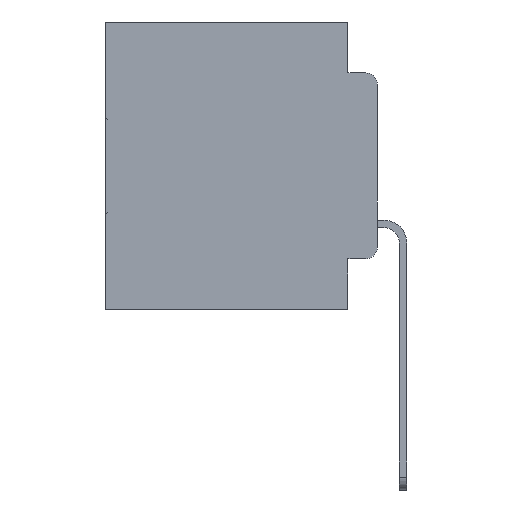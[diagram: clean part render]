
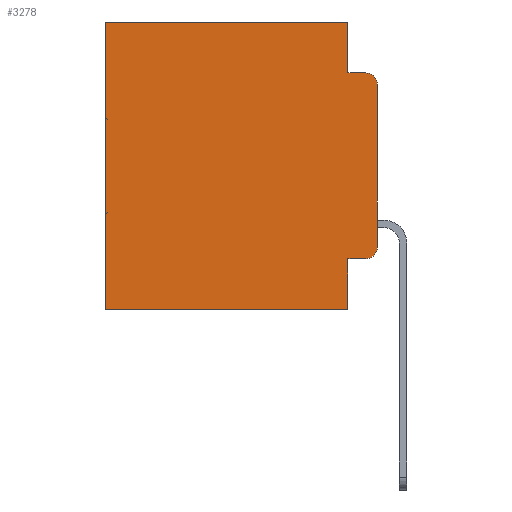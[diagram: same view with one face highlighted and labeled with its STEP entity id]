
A CAD part, left-side view. The second image highlights one B-rep face of the part: STEP entity #3278.
In plain terms, the highlighted planar face has unit normal (-1, 0, 0).
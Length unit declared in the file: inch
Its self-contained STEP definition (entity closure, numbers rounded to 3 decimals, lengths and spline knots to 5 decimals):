
#520 = DIRECTION ( 'NONE',  ( 0., 1., 0. ) ) ;
#866 = ORIENTED_EDGE ( 'NONE', *, *, #29314, .T. ) ;
#1343 = ORIENTED_EDGE ( 'NONE', *, *, #12030, .T. ) ;
#1952 = LINE ( 'NONE', #20739, #21634 ) ;
#2817 = CARTESIAN_POINT ( 'NONE',  ( 0.298, 0., 0. ) ) ;
#3278 = ADVANCED_FACE ( 'NONE', ( #25353 ), #19009, .F. ) ;
#3777 = CARTESIAN_POINT ( 'NONE',  ( 0.298, 0.02, -0.3915 ) ) ;
#4043 = ORIENTED_EDGE ( 'NONE', *, *, #12696, .F. ) ;
#4755 = ORIENTED_EDGE ( 'NONE', *, *, #29872, .F. ) ;
#5455 = CARTESIAN_POINT ( 'NONE',  ( 0.298, 0.051, 0. ) ) ;
#5644 = CARTESIAN_POINT ( 'NONE',  ( 0.298, 0.473, -0.5 ) ) ;
#6081 = VECTOR ( 'NONE', #30742, 39.37008 ) ;
#6240 = CARTESIAN_POINT ( 'NONE',  ( 0.298, 0., 0. ) ) ;
#6361 = DIRECTION ( 'NONE',  ( 0., 0., -1. ) ) ;
#6434 = LINE ( 'NONE', #2817, #7291 ) ;
#6481 = DIRECTION ( 'NONE',  ( 0., 0., -1. ) ) ;
#6741 = LINE ( 'NONE', #5455, #20157 ) ;
#7291 = VECTOR ( 'NONE', #20728, 39.37008 ) ;
#7894 = VERTEX_POINT ( 'NONE', #5644 ) ;
#8541 = VERTEX_POINT ( 'NONE', #19485 ) ;
#9896 = ORIENTED_EDGE ( 'NONE', *, *, #18399, .F. ) ;
#10313 = ORIENTED_EDGE ( 'NONE', *, *, #21648, .F. ) ;
#11189 = EDGE_CURVE ( 'NONE', #12075, #28483, #6434, .T. ) ;
#11825 = AXIS2_PLACEMENT_3D ( 'NONE', #6240, #21447, #6361 ) ;
#12024 = CARTESIAN_POINT ( 'NONE',  ( 0.298, 0.02, -0.1085 ) ) ;
#12030 = EDGE_CURVE ( 'NONE', #28483, #7894, #20564, .T. ) ;
#12075 = VERTEX_POINT ( 'NONE', #19070 ) ;
#12534 = LINE ( 'NONE', #13704, #31058 ) ;
#12696 = EDGE_CURVE ( 'NONE', #20193, #7894, #16787, .T. ) ;
#13370 = CARTESIAN_POINT ( 'NONE',  ( 0.298, 0.051, -0.5 ) ) ;
#13704 = CARTESIAN_POINT ( 'NONE',  ( 0.298, 0.051, 0. ) ) ;
#13837 = LINE ( 'NONE', #28328, #6081 ) ;
#14488 = DIRECTION ( 'NONE',  ( 0., 0., -1. ) ) ;
#14734 = EDGE_LOOP ( 'NONE', ( #27144, #866, #9896, #10313, #32414, #1343, #4043, #4755, #22200, #31221 ) ) ;
#15334 = EDGE_CURVE ( 'NONE', #8541, #15939, #1952, .T. ) ;
#15595 = VECTOR ( 'NONE', #18859, 39.37008 ) ;
#15907 = CARTESIAN_POINT ( 'NONE',  ( 0.298, 0.02, -0.0885 ) ) ;
#15939 = VERTEX_POINT ( 'NONE', #27233 ) ;
#16166 = DIRECTION ( 'NONE',  ( 0., 0., -1. ) ) ;
#16174 = VERTEX_POINT ( 'NONE', #15907 ) ;
#16417 = CARTESIAN_POINT ( 'NONE',  ( 0.298, 0.473, 0. ) ) ;
#16787 = LINE ( 'NONE', #21247, #28876 ) ;
#18399 = EDGE_CURVE ( 'NONE', #23174, #16174, #21355, .T. ) ;
#18656 = CARTESIAN_POINT ( 'NONE',  ( 0.298, 0.051, -0.4115 ) ) ;
#18859 = DIRECTION ( 'NONE',  ( 0., 0., -1. ) ) ;
#19009 = PLANE ( 'NONE',  #11825 ) ;
#19070 = CARTESIAN_POINT ( 'NONE',  ( 0.298, 0.051, 0. ) ) ;
#19485 = CARTESIAN_POINT ( 'NONE',  ( 0.298, 0., -0.1085 ) ) ;
#20157 = VECTOR ( 'NONE', #25492, 39.37008 ) ;
#20193 = VERTEX_POINT ( 'NONE', #13370 ) ;
#20564 = LINE ( 'NONE', #16417, #15595 ) ;
#20728 = DIRECTION ( 'NONE',  ( 0., 1., 0. ) ) ;
#20739 = CARTESIAN_POINT ( 'NONE',  ( 0.298, 0., 0. ) ) ;
#20946 = CIRCLE ( 'NONE', #25904, 0.02 ) ;
#21247 = CARTESIAN_POINT ( 'NONE',  ( 0.298, 0., -0.5 ) ) ;
#21355 = LINE ( 'NONE', #26623, #27022 ) ;
#21447 = DIRECTION ( 'NONE',  ( 1., 0., 0. ) ) ;
#21541 = DIRECTION ( 'NONE',  ( -1., 0., 0. ) ) ;
#21634 = VECTOR ( 'NONE', #23190, 39.37008 ) ;
#21648 = EDGE_CURVE ( 'NONE', #12075, #23174, #6741, .T. ) ;
#21872 = CARTESIAN_POINT ( 'NONE',  ( 0.298, 0.473, 0. ) ) ;
#22200 = ORIENTED_EDGE ( 'NONE', *, *, #25479, .T. ) ;
#22684 = CIRCLE ( 'NONE', #23071, 0.02 ) ;
#23071 = AXIS2_PLACEMENT_3D ( 'NONE', #3777, #21541, #6481 ) ;
#23174 = VERTEX_POINT ( 'NONE', #29600 ) ;
#23190 = DIRECTION ( 'NONE',  ( 0., 0., -1. ) ) ;
#23431 = CARTESIAN_POINT ( 'NONE',  ( 0.298, 0.02, -0.4115 ) ) ;
#24408 = EDGE_CURVE ( 'NONE', #29079, #15939, #22684, .T. ) ;
#25353 = FACE_OUTER_BOUND ( 'NONE', #14734, .T. ) ;
#25479 = EDGE_CURVE ( 'NONE', #29108, #29079, #13837, .T. ) ;
#25492 = DIRECTION ( 'NONE',  ( 0., 0., -1. ) ) ;
#25904 = AXIS2_PLACEMENT_3D ( 'NONE', #12024, #28986, #14488 ) ;
#26623 = CARTESIAN_POINT ( 'NONE',  ( 0.298, 0.051, -0.0885 ) ) ;
#26727 = DIRECTION ( 'NONE',  ( 0., -1., 0. ) ) ;
#27022 = VECTOR ( 'NONE', #26727, 39.37008 ) ;
#27144 = ORIENTED_EDGE ( 'NONE', *, *, #15334, .F. ) ;
#27233 = CARTESIAN_POINT ( 'NONE',  ( 0.298, 0., -0.3915 ) ) ;
#28328 = CARTESIAN_POINT ( 'NONE',  ( 0.298, 0.051, -0.4115 ) ) ;
#28483 = VERTEX_POINT ( 'NONE', #21872 ) ;
#28876 = VECTOR ( 'NONE', #520, 39.37008 ) ;
#28986 = DIRECTION ( 'NONE',  ( -1., 0., 0. ) ) ;
#29079 = VERTEX_POINT ( 'NONE', #23431 ) ;
#29108 = VERTEX_POINT ( 'NONE', #18656 ) ;
#29314 = EDGE_CURVE ( 'NONE', #8541, #16174, #20946, .T. ) ;
#29600 = CARTESIAN_POINT ( 'NONE',  ( 0.298, 0.051, -0.0885 ) ) ;
#29872 = EDGE_CURVE ( 'NONE', #29108, #20193, #12534, .T. ) ;
#30742 = DIRECTION ( 'NONE',  ( 0., -1., 0. ) ) ;
#31058 = VECTOR ( 'NONE', #16166, 39.37008 ) ;
#31221 = ORIENTED_EDGE ( 'NONE', *, *, #24408, .T. ) ;
#32414 = ORIENTED_EDGE ( 'NONE', *, *, #11189, .T. ) ;
